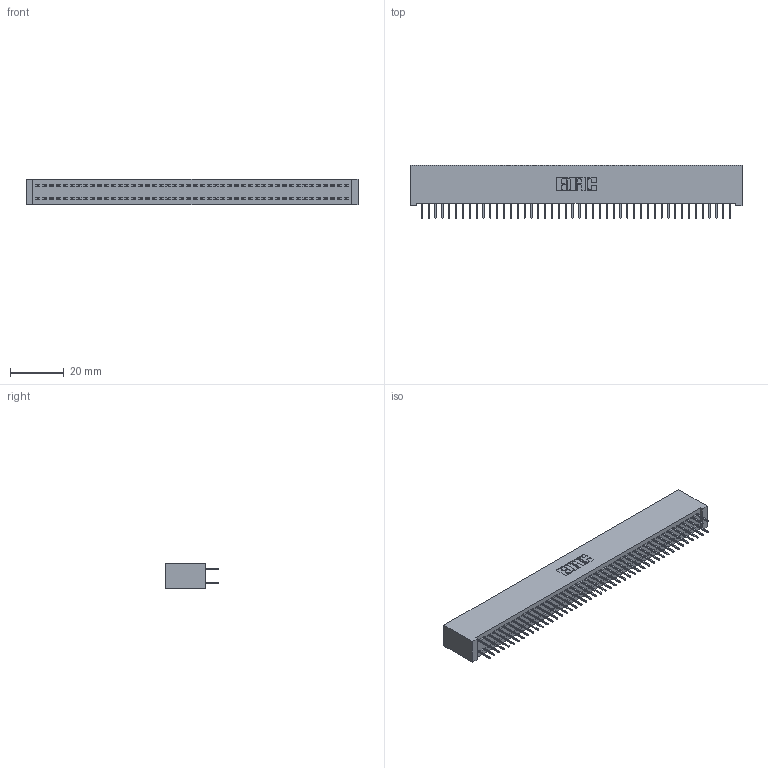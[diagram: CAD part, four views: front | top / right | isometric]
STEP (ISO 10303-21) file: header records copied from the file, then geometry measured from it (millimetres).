
FILE_DESCRIPTION (( 'STEP AP203' ), '1' );
FILE_NAME ('342-092-524-201.STEP', '2019-10-04T14:46:16', ( '' ), ( '' ), 'SwSTEP 2.0', 'SolidWorks 2016', '' );
FILE_SCHEMA (( 'CONFIG_CONTROL_DESIGN' ));
Length unit declared in the file: inch
Products named in the file (3): 342 Part_Lugless; 345-292-001_345-293-124; 342-092-524-201
Assembly tree (93 placements, depth 2):
  342-092-524-201
    342 Part_Lugless
    345-292-001_345-293-124  x92
Bounding box: 123.09 x 19.69 x 9.4 mm (x, y, z)
Volume: 11378.7 mm3; surface area: 18704.3 mm2
Topology: 93 solids, 93 shells, 5254 faces, 14903 edges, 9566 vertices
Faces by surface type: plane 3926, cylinder 1328
Entity records: 28741 total; most frequent: CARTESIAN_POINT 4754, ORIENTED_EDGE 4690, DIRECTION 4049, EDGE_CURVE 2345, VECTOR 2229, LINE 2229, VERTEX_POINT 1558, AXIS2_PLACEMENT_3D 910
